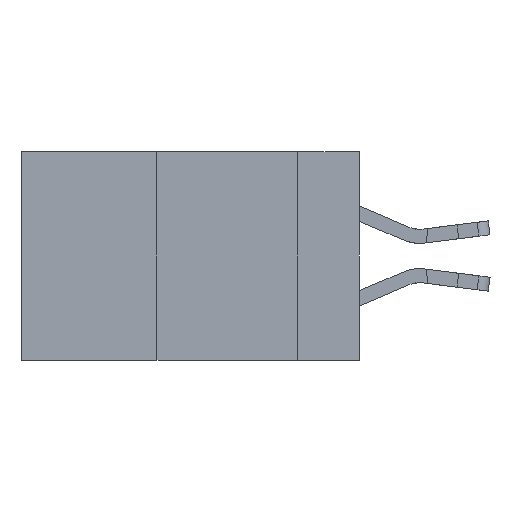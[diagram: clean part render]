
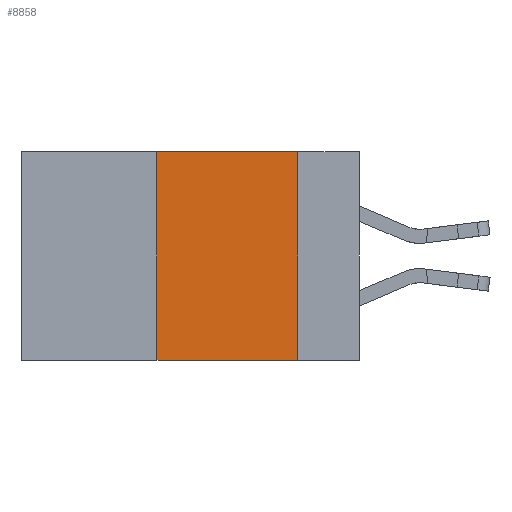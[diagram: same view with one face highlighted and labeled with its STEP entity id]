
A CAD part, left-side view. The second image highlights one B-rep face of the part: STEP entity #8858.
In plain terms, the highlighted planar face has unit normal (-1, 0, 0).
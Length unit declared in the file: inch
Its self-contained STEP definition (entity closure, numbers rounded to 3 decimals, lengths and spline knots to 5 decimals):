
#563 = CARTESIAN_POINT ( 'NONE',  ( 0., 0.36, 0. ) ) ;
#1683 = EDGE_CURVE ( 'NONE', #15242, #4032, #4211, .T. ) ;
#1848 = CARTESIAN_POINT ( 'NONE',  ( 0., 0.11, 0. ) ) ;
#2479 = ORIENTED_EDGE ( 'NONE', *, *, #1683, .F. ) ;
#4032 = VERTEX_POINT ( 'NONE', #10251 ) ;
#4211 = LINE ( 'NONE', #7774, #8760 ) ;
#6353 = CARTESIAN_POINT ( 'NONE',  ( 0., 0.36, 0. ) ) ;
#7774 = CARTESIAN_POINT ( 'NONE',  ( 0., 0.11, 0. ) ) ;
#8240 = DIRECTION ( 'NONE',  ( 0., 0., -1. ) ) ;
#8355 = FACE_OUTER_BOUND ( 'NONE', #20270, .T. ) ;
#8370 = VECTOR ( 'NONE', #10486, 39.37008 ) ;
#8760 = VECTOR ( 'NONE', #27182, 39.37008 ) ;
#8858 = ADVANCED_FACE ( 'NONE', ( #8355 ), #22280, .F. ) ;
#9340 = ORIENTED_EDGE ( 'NONE', *, *, #21176, .F. ) ;
#10251 = CARTESIAN_POINT ( 'NONE',  ( 0., 0.11, -0.37 ) ) ;
#10462 = DIRECTION ( 'NONE',  ( 1., 0., 0. ) ) ;
#10486 = DIRECTION ( 'NONE',  ( 0., -1., 0. ) ) ;
#10989 = AXIS2_PLACEMENT_3D ( 'NONE', #29703, #10462, #8240 ) ;
#12127 = VERTEX_POINT ( 'NONE', #14360 ) ;
#12586 = EDGE_CURVE ( 'NONE', #12127, #4032, #26809, .T. ) ;
#14360 = CARTESIAN_POINT ( 'NONE',  ( 0., 0.36, -0.37 ) ) ;
#15242 = VERTEX_POINT ( 'NONE', #1848 ) ;
#15491 = CARTESIAN_POINT ( 'NONE',  ( 0., 0.6, 0. ) ) ;
#18180 = ORIENTED_EDGE ( 'NONE', *, *, #22642, .F. ) ;
#20270 = EDGE_LOOP ( 'NONE', ( #2479, #9340, #18180, #30898 ) ) ;
#21176 = EDGE_CURVE ( 'NONE', #27448, #15242, #22435, .T. ) ;
#21504 = DIRECTION ( 'NONE',  ( 0., -1., 0. ) ) ;
#22280 = PLANE ( 'NONE',  #10989 ) ;
#22435 = LINE ( 'NONE', #15491, #8370 ) ;
#22642 = EDGE_CURVE ( 'NONE', #12127, #27448, #26162, .T. ) ;
#26162 = LINE ( 'NONE', #563, #27259 ) ;
#26809 = LINE ( 'NONE', #30571, #28703 ) ;
#26991 = DIRECTION ( 'NONE',  ( 0., 0., 1. ) ) ;
#27182 = DIRECTION ( 'NONE',  ( 0., 0., -1. ) ) ;
#27259 = VECTOR ( 'NONE', #26991, 39.37008 ) ;
#27448 = VERTEX_POINT ( 'NONE', #6353 ) ;
#28703 = VECTOR ( 'NONE', #21504, 39.37008 ) ;
#29703 = CARTESIAN_POINT ( 'NONE',  ( 0., 0.6, 0. ) ) ;
#30571 = CARTESIAN_POINT ( 'NONE',  ( 0., 0.6, -0.37 ) ) ;
#30898 = ORIENTED_EDGE ( 'NONE', *, *, #12586, .T. ) ;
